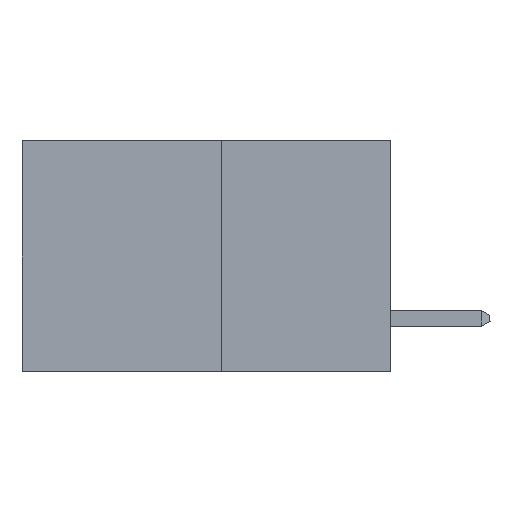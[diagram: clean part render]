
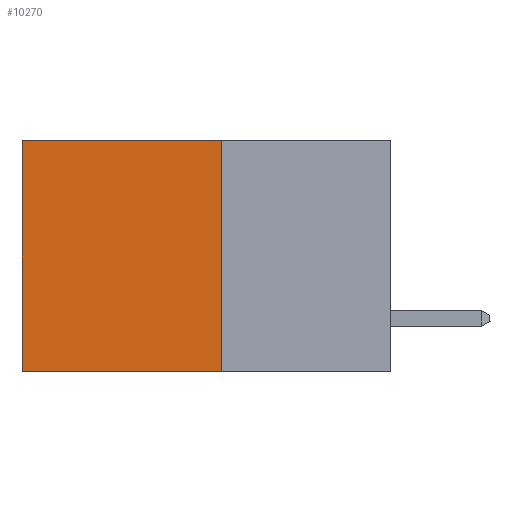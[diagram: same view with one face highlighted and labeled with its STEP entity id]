
A CAD part, left-side view. The second image highlights one B-rep face of the part: STEP entity #10270.
In plain terms, the highlighted planar face has unit normal (-1, 0, 0).
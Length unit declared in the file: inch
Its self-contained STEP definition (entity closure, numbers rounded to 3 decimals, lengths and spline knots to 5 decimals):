
#343 = EDGE_CURVE ( 'NONE', #3582, #19289, #17893, .T. ) ;
#565 = LINE ( 'NONE', #17014, #14009 ) ;
#1851 = PLANE ( 'NONE',  #9230 ) ;
#2721 = FACE_OUTER_BOUND ( 'NONE', #7675, .T. ) ;
#3467 = CARTESIAN_POINT ( 'NONE',  ( 0.277, 0.59, 0. ) ) ;
#3582 = VERTEX_POINT ( 'NONE', #14888 ) ;
#4246 = EDGE_CURVE ( 'NONE', #10822, #18482, #7208, .T. ) ;
#4757 = LINE ( 'NONE', #9217, #12500 ) ;
#5076 = DIRECTION ( 'NONE',  ( 0., 0., -1. ) ) ;
#5725 = CARTESIAN_POINT ( 'NONE',  ( 0.277, 0.59, -0.37 ) ) ;
#6583 = CARTESIAN_POINT ( 'NONE',  ( 0.277, 0.59, -0.37 ) ) ;
#6733 = DIRECTION ( 'NONE',  ( 0., 0., -1. ) ) ;
#6752 = DIRECTION ( 'NONE',  ( 0., 0., -1. ) ) ;
#7208 = LINE ( 'NONE', #6583, #14907 ) ;
#7675 = EDGE_LOOP ( 'NONE', ( #11969, #9400, #15446, #13648 ) ) ;
#8623 = EDGE_CURVE ( 'NONE', #3582, #10822, #4757, .T. ) ;
#9217 = CARTESIAN_POINT ( 'NONE',  ( 0.277, 0.27, 0. ) ) ;
#9230 = AXIS2_PLACEMENT_3D ( 'NONE', #12770, #14307, #5076 ) ;
#9400 = ORIENTED_EDGE ( 'NONE', *, *, #16580, .F. ) ;
#10270 = ADVANCED_FACE ( 'NONE', ( #2721 ), #1851, .F. ) ;
#10822 = VERTEX_POINT ( 'NONE', #3467 ) ;
#10898 = DIRECTION ( 'NONE',  ( 0., 1., 0. ) ) ;
#11090 = CARTESIAN_POINT ( 'NONE',  ( 0.277, 0.27, -0.37 ) ) ;
#11969 = ORIENTED_EDGE ( 'NONE', *, *, #4246, .T. ) ;
#12500 = VECTOR ( 'NONE', #13883, 39.37008 ) ;
#12770 = CARTESIAN_POINT ( 'NONE',  ( 0.277, 0.27, -0.37 ) ) ;
#12900 = CARTESIAN_POINT ( 'NONE',  ( 0.277, 0.27, -0.37 ) ) ;
#13648 = ORIENTED_EDGE ( 'NONE', *, *, #8623, .T. ) ;
#13883 = DIRECTION ( 'NONE',  ( 0., 1., 0. ) ) ;
#13886 = VECTOR ( 'NONE', #6733, 39.37008 ) ;
#14009 = VECTOR ( 'NONE', #10898, 39.37008 ) ;
#14307 = DIRECTION ( 'NONE',  ( 1., 0., 0. ) ) ;
#14888 = CARTESIAN_POINT ( 'NONE',  ( 0.277, 0.27, 0. ) ) ;
#14907 = VECTOR ( 'NONE', #6752, 39.37008 ) ;
#15446 = ORIENTED_EDGE ( 'NONE', *, *, #343, .F. ) ;
#16580 = EDGE_CURVE ( 'NONE', #19289, #18482, #565, .T. ) ;
#17014 = CARTESIAN_POINT ( 'NONE',  ( 0.277, 0.27, -0.37 ) ) ;
#17893 = LINE ( 'NONE', #12900, #13886 ) ;
#18482 = VERTEX_POINT ( 'NONE', #5725 ) ;
#19289 = VERTEX_POINT ( 'NONE', #11090 ) ;
